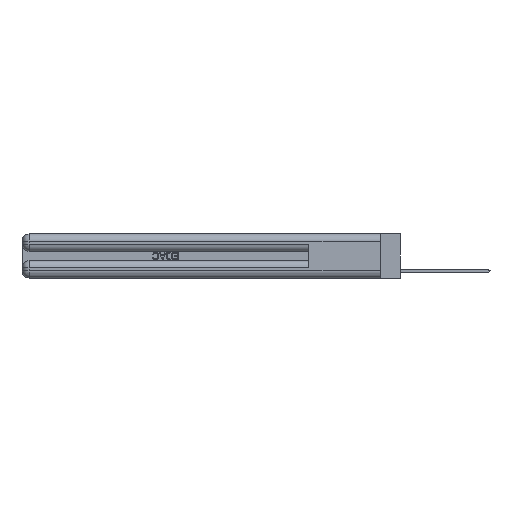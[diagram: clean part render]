
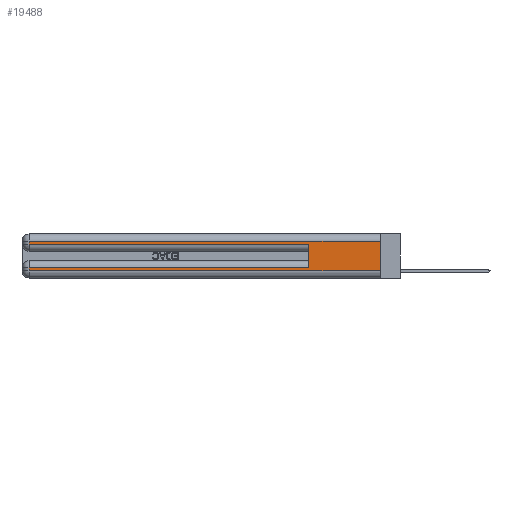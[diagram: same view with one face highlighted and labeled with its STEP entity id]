
A CAD part, left-side view. The second image highlights one B-rep face of the part: STEP entity #19488.
In plain terms, the highlighted planar face has unit normal (-1, 0, 0).
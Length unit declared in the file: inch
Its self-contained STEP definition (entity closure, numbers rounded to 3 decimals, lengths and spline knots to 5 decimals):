
#337 = AXIS2_PLACEMENT_3D ( 'NONE', #2008, #21926, #21781 ) ;
#1571 = CARTESIAN_POINT ( 'NONE',  ( 0., 0., 0.31 ) ) ;
#1576 = CARTESIAN_POINT ( 'NONE',  ( 0., 2.94, 0.37 ) ) ;
#2008 = CARTESIAN_POINT ( 'NONE',  ( 0., 0., 0.37 ) ) ;
#2168 = VERTEX_POINT ( 'NONE', #3332 ) ;
#2221 = CARTESIAN_POINT ( 'NONE',  ( 0., 2.94, 0.06 ) ) ;
#2526 = LINE ( 'NONE', #5441, #5916 ) ;
#3332 = CARTESIAN_POINT ( 'NONE',  ( 0., 0.6, 0.285 ) ) ;
#3550 = EDGE_CURVE ( 'NONE', #13125, #8274, #9602, .T. ) ;
#3878 = VECTOR ( 'NONE', #27855, 39.37008 ) ;
#4163 = DIRECTION ( 'NONE',  ( 0., 0., -1. ) ) ;
#4477 = EDGE_CURVE ( 'NONE', #8274, #6817, #2526, .T. ) ;
#5042 = DIRECTION ( 'NONE',  ( 0., 0., -1. ) ) ;
#5441 = CARTESIAN_POINT ( 'NONE',  ( 0., 2.94, 0.37 ) ) ;
#5916 = VECTOR ( 'NONE', #5042, 39.37008 ) ;
#6817 = VERTEX_POINT ( 'NONE', #2221 ) ;
#7031 = EDGE_CURVE ( 'NONE', #11618, #26688, #14628, .T. ) ;
#7542 = ORIENTED_EDGE ( 'NONE', *, *, #4477, .T. ) ;
#7963 = ORIENTED_EDGE ( 'NONE', *, *, #3550, .T. ) ;
#8274 = VERTEX_POINT ( 'NONE', #13967 ) ;
#8338 = EDGE_CURVE ( 'NONE', #12106, #11618, #25700, .T. ) ;
#9602 = LINE ( 'NONE', #16236, #17114 ) ;
#10310 = CARTESIAN_POINT ( 'NONE',  ( 0., 0., 0.37 ) ) ;
#10574 = VERTEX_POINT ( 'NONE', #26446 ) ;
#10623 = LINE ( 'NONE', #28335, #16018 ) ;
#10801 = EDGE_CURVE ( 'NONE', #26688, #2168, #26418, .T. ) ;
#11049 = ORIENTED_EDGE ( 'NONE', *, *, #7031, .T. ) ;
#11618 = VERTEX_POINT ( 'NONE', #21844 ) ;
#12106 = VERTEX_POINT ( 'NONE', #1571 ) ;
#12109 = DIRECTION ( 'NONE',  ( 0., 1., 0. ) ) ;
#12694 = FACE_OUTER_BOUND ( 'NONE', #14785, .T. ) ;
#12973 = DIRECTION ( 'NONE',  ( 0., 0., -1. ) ) ;
#13125 = VERTEX_POINT ( 'NONE', #14387 ) ;
#13967 = CARTESIAN_POINT ( 'NONE',  ( 0., 2.94, 0.085 ) ) ;
#14387 = CARTESIAN_POINT ( 'NONE',  ( 0., 0.6, 0.085 ) ) ;
#14628 = LINE ( 'NONE', #1576, #27826 ) ;
#14785 = EDGE_LOOP ( 'NONE', ( #16577, #22217, #11049, #18297, #17760, #7963, #7542, #25834 ) ) ;
#15195 = PLANE ( 'NONE',  #337 ) ;
#16018 = VECTOR ( 'NONE', #26289, 39.37008 ) ;
#16236 = CARTESIAN_POINT ( 'NONE',  ( 0., 0., 0.085 ) ) ;
#16577 = ORIENTED_EDGE ( 'NONE', *, *, #23764, .F. ) ;
#17114 = VECTOR ( 'NONE', #12109, 39.37008 ) ;
#17444 = CARTESIAN_POINT ( 'NONE',  ( 0., 2.94, 0.285 ) ) ;
#17632 = DIRECTION ( 'NONE',  ( 0., -1., 0. ) ) ;
#17760 = ORIENTED_EDGE ( 'NONE', *, *, #25850, .F. ) ;
#18297 = ORIENTED_EDGE ( 'NONE', *, *, #10801, .T. ) ;
#18648 = LINE ( 'NONE', #25675, #3878 ) ;
#18952 = CARTESIAN_POINT ( 'NONE',  ( 0., 0., 0.31 ) ) ;
#19488 = ADVANCED_FACE ( 'NONE', ( #12694 ), #15195, .F. ) ;
#21001 = DIRECTION ( 'NONE',  ( 0., 1., 0. ) ) ;
#21781 = DIRECTION ( 'NONE',  ( 0., 0., -1. ) ) ;
#21844 = CARTESIAN_POINT ( 'NONE',  ( 0., 2.94, 0.31 ) ) ;
#21926 = DIRECTION ( 'NONE',  ( 1., 0., 0. ) ) ;
#22217 = ORIENTED_EDGE ( 'NONE', *, *, #8338, .T. ) ;
#23764 = EDGE_CURVE ( 'NONE', #12106, #10574, #26137, .T. ) ;
#24317 = VECTOR ( 'NONE', #4163, 39.37008 ) ;
#24722 = VECTOR ( 'NONE', #17632, 39.37008 ) ;
#25658 = VECTOR ( 'NONE', #21001, 39.37008 ) ;
#25675 = CARTESIAN_POINT ( 'NONE',  ( 0., 0., 0.06 ) ) ;
#25700 = LINE ( 'NONE', #18952, #25658 ) ;
#25834 = ORIENTED_EDGE ( 'NONE', *, *, #27183, .T. ) ;
#25850 = EDGE_CURVE ( 'NONE', #13125, #2168, #10623, .T. ) ;
#26137 = LINE ( 'NONE', #10310, #24317 ) ;
#26289 = DIRECTION ( 'NONE',  ( 0., 0., 1. ) ) ;
#26418 = LINE ( 'NONE', #26710, #24722 ) ;
#26446 = CARTESIAN_POINT ( 'NONE',  ( 0., 0., 0.06 ) ) ;
#26688 = VERTEX_POINT ( 'NONE', #17444 ) ;
#26710 = CARTESIAN_POINT ( 'NONE',  ( 0., 0., 0.285 ) ) ;
#27183 = EDGE_CURVE ( 'NONE', #6817, #10574, #18648, .T. ) ;
#27826 = VECTOR ( 'NONE', #12973, 39.37008 ) ;
#27855 = DIRECTION ( 'NONE',  ( 0., -1., 0. ) ) ;
#28335 = CARTESIAN_POINT ( 'NONE',  ( 0., 0.6, 0.145 ) ) ;
